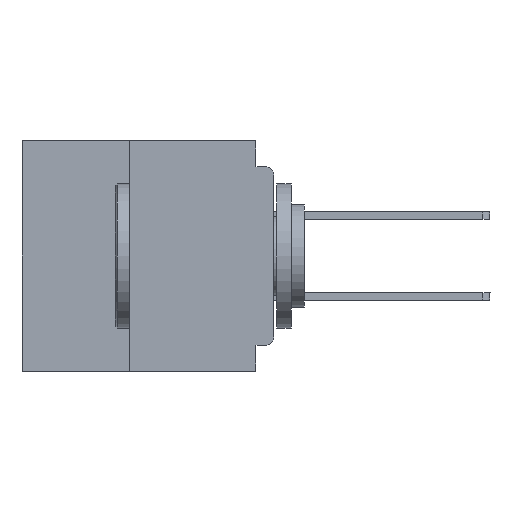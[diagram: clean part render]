
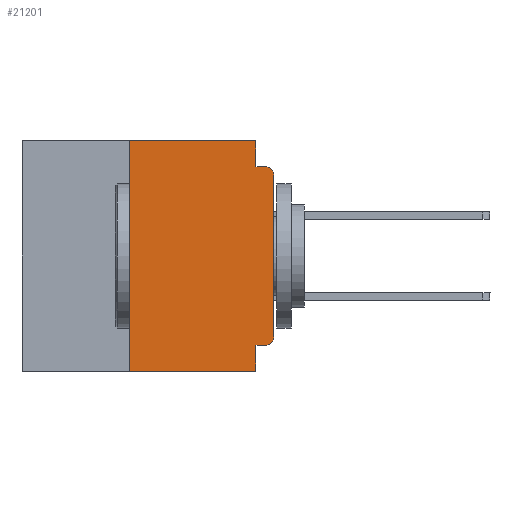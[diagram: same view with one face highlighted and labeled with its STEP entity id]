
A CAD part, left-side view. The second image highlights one B-rep face of the part: STEP entity #21201.
In plain terms, the highlighted planar face has unit normal (-1, 0, 0).
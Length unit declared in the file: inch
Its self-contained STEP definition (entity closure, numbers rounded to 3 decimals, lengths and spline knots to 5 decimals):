
#785 = DIRECTION ( 'NONE',  ( 0., 0., -1. ) ) ;
#1953 = VECTOR ( 'NONE', #37932, 39.37008 ) ;
#2660 = VECTOR ( 'NONE', #20851, 39.37008 ) ;
#3460 = CIRCLE ( 'NONE', #23377, 0.015 ) ;
#4094 = LINE ( 'NONE', #11021, #55031 ) ;
#4733 = EDGE_LOOP ( 'NONE', ( #58660, #28010, #20371, #24400, #12974, #61131, #28215, #47950, #56193, #47214 ) ) ;
#7416 = CARTESIAN_POINT ( 'NONE',  ( 0., 0.25, 0. ) ) ;
#9380 = DIRECTION ( 'NONE',  ( -1., 0., 0. ) ) ;
#10772 = DIRECTION ( 'NONE',  ( 0., 0., -1. ) ) ;
#11021 = CARTESIAN_POINT ( 'NONE',  ( 0., 0.437, 0. ) ) ;
#11259 = PLANE ( 'NONE',  #61477 ) ;
#12178 = CARTESIAN_POINT ( 'NONE',  ( 0., 0.015, -0.045 ) ) ;
#12529 = EDGE_CURVE ( 'NONE', #40758, #29648, #3460, .T. ) ;
#12719 = EDGE_CURVE ( 'NONE', #31526, #55253, #15836, .T. ) ;
#12974 = ORIENTED_EDGE ( 'NONE', *, *, #16948, .F. ) ;
#13215 = CARTESIAN_POINT ( 'NONE',  ( 0., 0.437, -0.4 ) ) ;
#14112 = CARTESIAN_POINT ( 'NONE',  ( 0., 0., -0.045 ) ) ;
#14277 = VERTEX_POINT ( 'NONE', #7416 ) ;
#14477 = DIRECTION ( 'NONE',  ( 0., 0., -1. ) ) ;
#15836 = LINE ( 'NONE', #40558, #2660 ) ;
#16611 = LINE ( 'NONE', #40426, #34483 ) ;
#16687 = AXIS2_PLACEMENT_3D ( 'NONE', #59822, #30507, #785 ) ;
#16928 = LINE ( 'NONE', #42564, #54700 ) ;
#16948 = EDGE_CURVE ( 'NONE', #14277, #24294, #4094, .T. ) ;
#16985 = CARTESIAN_POINT ( 'NONE',  ( 0., 0.25, -0.4 ) ) ;
#17813 = CARTESIAN_POINT ( 'NONE',  ( 0., 0.031, -0.4 ) ) ;
#20371 = ORIENTED_EDGE ( 'NONE', *, *, #33342, .F. ) ;
#20517 = VECTOR ( 'NONE', #43769, 39.37008 ) ;
#20851 = DIRECTION ( 'NONE',  ( 0., 1., 0. ) ) ;
#21201 = ADVANCED_FACE ( 'NONE', ( #46495 ), #11259, .F. ) ;
#21218 = DIRECTION ( 'NONE',  ( 0., 0., -1. ) ) ;
#23377 = AXIS2_PLACEMENT_3D ( 'NONE', #39100, #9380, #44037 ) ;
#23642 = LINE ( 'NONE', #14112, #20517 ) ;
#24294 = VERTEX_POINT ( 'NONE', #28206 ) ;
#24400 = ORIENTED_EDGE ( 'NONE', *, *, #58140, .F. ) ;
#25714 = CARTESIAN_POINT ( 'NONE',  ( 0., 0., -0.06 ) ) ;
#27848 = DIRECTION ( 'NONE',  ( 0., 0., 1. ) ) ;
#28010 = ORIENTED_EDGE ( 'NONE', *, *, #12529, .T. ) ;
#28206 = CARTESIAN_POINT ( 'NONE',  ( 0., 0.031, 0. ) ) ;
#28215 = ORIENTED_EDGE ( 'NONE', *, *, #59792, .T. ) ;
#29648 = VERTEX_POINT ( 'NONE', #12178 ) ;
#30507 = DIRECTION ( 'NONE',  ( -1., 0., 0. ) ) ;
#31526 = VERTEX_POINT ( 'NONE', #32783 ) ;
#32783 = CARTESIAN_POINT ( 'NONE',  ( 0., 0.015, -0.355 ) ) ;
#33342 = EDGE_CURVE ( 'NONE', #60348, #29648, #23642, .T. ) ;
#33938 = CARTESIAN_POINT ( 'NONE',  ( 0., 0., -0.34 ) ) ;
#34219 = CARTESIAN_POINT ( 'NONE',  ( 0., 0.031, 0. ) ) ;
#34483 = VECTOR ( 'NONE', #10772, 39.37008 ) ;
#35537 = LINE ( 'NONE', #34219, #59987 ) ;
#37439 = CARTESIAN_POINT ( 'NONE',  ( 0., 0.031, -0.045 ) ) ;
#37932 = DIRECTION ( 'NONE',  ( 0., -1., 0. ) ) ;
#39100 = CARTESIAN_POINT ( 'NONE',  ( 0., 0.015, -0.06 ) ) ;
#40426 = CARTESIAN_POINT ( 'NONE',  ( 0., 0.031, -0.4 ) ) ;
#40558 = CARTESIAN_POINT ( 'NONE',  ( 0., 0., -0.355 ) ) ;
#40667 = DIRECTION ( 'NONE',  ( 0., -1., 0. ) ) ;
#40692 = EDGE_CURVE ( 'NONE', #31526, #46783, #55324, .T. ) ;
#40758 = VERTEX_POINT ( 'NONE', #25714 ) ;
#41208 = CARTESIAN_POINT ( 'NONE',  ( 0., 0.25, -0.4 ) ) ;
#42564 = CARTESIAN_POINT ( 'NONE',  ( 0., 0., 0. ) ) ;
#43769 = DIRECTION ( 'NONE',  ( 0., -1., 0. ) ) ;
#44037 = DIRECTION ( 'NONE',  ( 0., 0., -1. ) ) ;
#44413 = VERTEX_POINT ( 'NONE', #16985 ) ;
#45853 = CARTESIAN_POINT ( 'NONE',  ( 0., 0.437, 0. ) ) ;
#46183 = DIRECTION ( 'NONE',  ( 0., 0., 1. ) ) ;
#46495 = FACE_OUTER_BOUND ( 'NONE', #4733, .T. ) ;
#46783 = VERTEX_POINT ( 'NONE', #33938 ) ;
#47026 = CARTESIAN_POINT ( 'NONE',  ( 0., 0.031, -0.355 ) ) ;
#47214 = ORIENTED_EDGE ( 'NONE', *, *, #40692, .T. ) ;
#47950 = ORIENTED_EDGE ( 'NONE', *, *, #52660, .F. ) ;
#49618 = VECTOR ( 'NONE', #46183, 39.37008 ) ;
#50782 = DIRECTION ( 'NONE',  ( 1., 0., 0. ) ) ;
#51147 = LINE ( 'NONE', #41208, #49618 ) ;
#52660 = EDGE_CURVE ( 'NONE', #55253, #62080, #16611, .T. ) ;
#54447 = LINE ( 'NONE', #13215, #1953 ) ;
#54700 = VECTOR ( 'NONE', #27848, 39.37008 ) ;
#55031 = VECTOR ( 'NONE', #40667, 39.37008 ) ;
#55147 = EDGE_CURVE ( 'NONE', #44413, #14277, #51147, .T. ) ;
#55253 = VERTEX_POINT ( 'NONE', #47026 ) ;
#55324 = CIRCLE ( 'NONE', #16687, 0.015 ) ;
#56193 = ORIENTED_EDGE ( 'NONE', *, *, #12719, .F. ) ;
#56505 = EDGE_CURVE ( 'NONE', #46783, #40758, #16928, .T. ) ;
#58140 = EDGE_CURVE ( 'NONE', #24294, #60348, #35537, .T. ) ;
#58660 = ORIENTED_EDGE ( 'NONE', *, *, #56505, .T. ) ;
#59792 = EDGE_CURVE ( 'NONE', #44413, #62080, #54447, .T. ) ;
#59822 = CARTESIAN_POINT ( 'NONE',  ( 0., 0.015, -0.34 ) ) ;
#59987 = VECTOR ( 'NONE', #14477, 39.37008 ) ;
#60348 = VERTEX_POINT ( 'NONE', #37439 ) ;
#61131 = ORIENTED_EDGE ( 'NONE', *, *, #55147, .F. ) ;
#61477 = AXIS2_PLACEMENT_3D ( 'NONE', #45853, #50782, #21218 ) ;
#62080 = VERTEX_POINT ( 'NONE', #17813 ) ;
